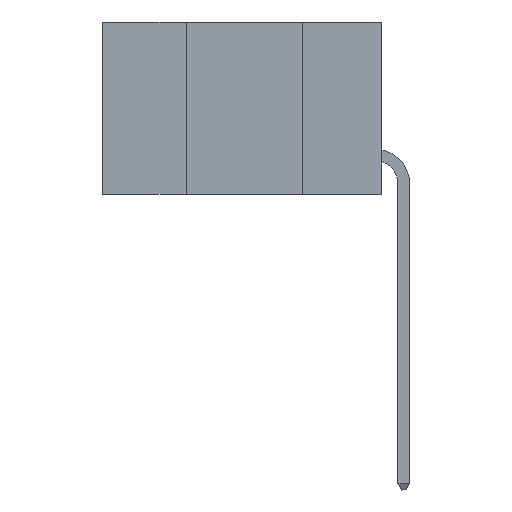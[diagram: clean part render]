
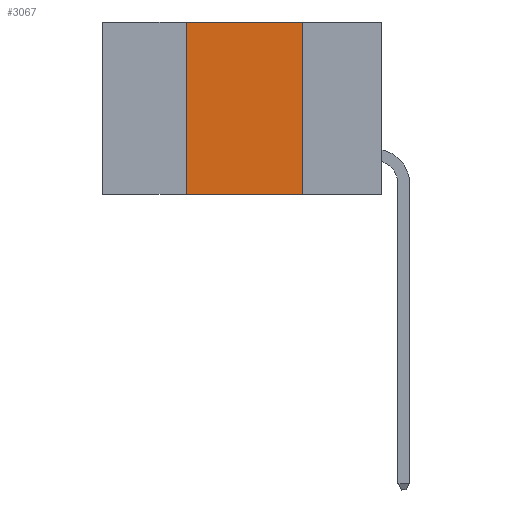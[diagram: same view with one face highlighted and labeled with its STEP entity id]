
A CAD part, left-side view. The second image highlights one B-rep face of the part: STEP entity #3067.
In plain terms, the highlighted planar face has unit normal (-1, 0, 0).
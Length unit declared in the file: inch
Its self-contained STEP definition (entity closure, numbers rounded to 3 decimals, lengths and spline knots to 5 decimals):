
#718 = AXIS2_PLACEMENT_3D ( 'NONE', #1486, #1416, #2267 ) ;
#946 = DIRECTION ( 'NONE',  ( 0., -1., 0. ) ) ;
#1376 = PLANE ( 'NONE',  #718 ) ;
#1416 = DIRECTION ( 'NONE',  ( 1., 0., 0. ) ) ;
#1486 = CARTESIAN_POINT ( 'NONE',  ( 0., 0.6, 0. ) ) ;
#1531 = CARTESIAN_POINT ( 'NONE',  ( 0., 0.17, -0.37 ) ) ;
#1685 = EDGE_CURVE ( 'NONE', #3790, #3116, #2487, .T. ) ;
#1758 = ORIENTED_EDGE ( 'NONE', *, *, #5226, .F. ) ;
#1821 = VERTEX_POINT ( 'NONE', #1936 ) ;
#1936 = CARTESIAN_POINT ( 'NONE',  ( 0., 0.42, -0.37 ) ) ;
#2267 = DIRECTION ( 'NONE',  ( 0., 0., -1. ) ) ;
#2487 = LINE ( 'NONE', #7534, #9021 ) ;
#3031 = DIRECTION ( 'NONE',  ( 0., -1., 0. ) ) ;
#3067 = ADVANCED_FACE ( 'NONE', ( #8316 ), #1376, .F. ) ;
#3116 = VERTEX_POINT ( 'NONE', #5568 ) ;
#3384 = ORIENTED_EDGE ( 'NONE', *, *, #1685, .F. ) ;
#3790 = VERTEX_POINT ( 'NONE', #6676 ) ;
#3858 = DIRECTION ( 'NONE',  ( 0., 0., -1. ) ) ;
#4093 = VECTOR ( 'NONE', #3858, 39.37008 ) ;
#4288 = LINE ( 'NONE', #8069, #9946 ) ;
#4309 = ORIENTED_EDGE ( 'NONE', *, *, #9256, .T. ) ;
#4504 = LINE ( 'NONE', #7975, #9211 ) ;
#5226 = EDGE_CURVE ( 'NONE', #1821, #3790, #4504, .T. ) ;
#5568 = CARTESIAN_POINT ( 'NONE',  ( 0., 0.17, 0. ) ) ;
#5757 = LINE ( 'NONE', #8721, #4093 ) ;
#6676 = CARTESIAN_POINT ( 'NONE',  ( 0., 0.42, 0. ) ) ;
#7320 = VERTEX_POINT ( 'NONE', #1531 ) ;
#7534 = CARTESIAN_POINT ( 'NONE',  ( 0., 0.6, 0. ) ) ;
#7782 = EDGE_CURVE ( 'NONE', #3116, #7320, #5757, .T. ) ;
#7950 = ORIENTED_EDGE ( 'NONE', *, *, #7782, .F. ) ;
#7975 = CARTESIAN_POINT ( 'NONE',  ( 0., 0.42, 0. ) ) ;
#8069 = CARTESIAN_POINT ( 'NONE',  ( 0., 0.6, -0.37 ) ) ;
#8316 = FACE_OUTER_BOUND ( 'NONE', #9473, .T. ) ;
#8721 = CARTESIAN_POINT ( 'NONE',  ( 0., 0.17, 0. ) ) ;
#9021 = VECTOR ( 'NONE', #946, 39.37008 ) ;
#9211 = VECTOR ( 'NONE', #10503, 39.37008 ) ;
#9256 = EDGE_CURVE ( 'NONE', #1821, #7320, #4288, .T. ) ;
#9473 = EDGE_LOOP ( 'NONE', ( #7950, #3384, #1758, #4309 ) ) ;
#9946 = VECTOR ( 'NONE', #3031, 39.37008 ) ;
#10503 = DIRECTION ( 'NONE',  ( 0., 0., 1. ) ) ;
